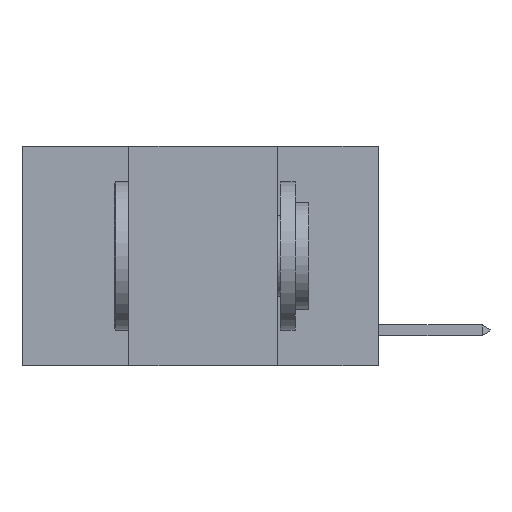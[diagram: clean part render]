
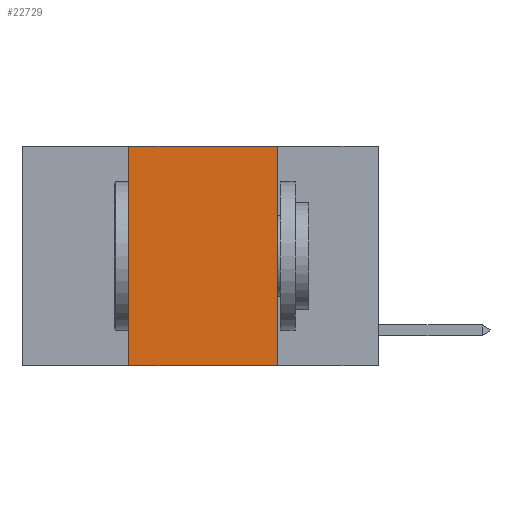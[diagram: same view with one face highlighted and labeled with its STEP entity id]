
A CAD part, left-side view. The second image highlights one B-rep face of the part: STEP entity #22729.
In plain terms, the highlighted planar face has unit normal (-1, 0, 0).
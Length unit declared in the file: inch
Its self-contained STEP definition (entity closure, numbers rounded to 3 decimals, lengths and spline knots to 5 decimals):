
#395 = DIRECTION ( 'NONE',  ( 0., 0., -1. ) ) ;
#428 = DIRECTION ( 'NONE',  ( 0., -1., 0. ) ) ;
#905 = VERTEX_POINT ( 'NONE', #9219 ) ;
#1697 = CARTESIAN_POINT ( 'NONE',  ( 0., 0.17, 0. ) ) ;
#2740 = VERTEX_POINT ( 'NONE', #23061 ) ;
#3685 = VECTOR ( 'NONE', #7489, 39.37008 ) ;
#4516 = PLANE ( 'NONE',  #23777 ) ;
#5400 = CARTESIAN_POINT ( 'NONE',  ( 0., 0.17, 0. ) ) ;
#5735 = ORIENTED_EDGE ( 'NONE', *, *, #16567, .F. ) ;
#7364 = DIRECTION ( 'NONE',  ( 0., -1., 0. ) ) ;
#7368 = ORIENTED_EDGE ( 'NONE', *, *, #22128, .T. ) ;
#7489 = DIRECTION ( 'NONE',  ( 0., 0., -1. ) ) ;
#9219 = CARTESIAN_POINT ( 'NONE',  ( 0., 0.17, -0.37 ) ) ;
#9378 = VECTOR ( 'NONE', #24487, 39.37008 ) ;
#10630 = VERTEX_POINT ( 'NONE', #1697 ) ;
#12193 = VERTEX_POINT ( 'NONE', #12789 ) ;
#12789 = CARTESIAN_POINT ( 'NONE',  ( 0., 0.42, -0.37 ) ) ;
#12941 = DIRECTION ( 'NONE',  ( 1., 0., 0. ) ) ;
#13678 = CARTESIAN_POINT ( 'NONE',  ( 0., 0.6, 0. ) ) ;
#15612 = LINE ( 'NONE', #22402, #9378 ) ;
#15742 = LINE ( 'NONE', #25429, #26122 ) ;
#16515 = ORIENTED_EDGE ( 'NONE', *, *, #19323, .F. ) ;
#16567 = EDGE_CURVE ( 'NONE', #10630, #905, #20302, .T. ) ;
#16672 = FACE_OUTER_BOUND ( 'NONE', #26459, .T. ) ;
#19323 = EDGE_CURVE ( 'NONE', #12193, #2740, #15612, .T. ) ;
#20302 = LINE ( 'NONE', #5400, #3685 ) ;
#22128 = EDGE_CURVE ( 'NONE', #12193, #905, #15742, .T. ) ;
#22402 = CARTESIAN_POINT ( 'NONE',  ( 0., 0.42, 0. ) ) ;
#22729 = ADVANCED_FACE ( 'NONE', ( #16672 ), #4516, .F. ) ;
#23061 = CARTESIAN_POINT ( 'NONE',  ( 0., 0.42, 0. ) ) ;
#23777 = AXIS2_PLACEMENT_3D ( 'NONE', #25398, #12941, #395 ) ;
#24321 = ORIENTED_EDGE ( 'NONE', *, *, #25746, .F. ) ;
#24487 = DIRECTION ( 'NONE',  ( 0., 0., 1. ) ) ;
#24615 = VECTOR ( 'NONE', #7364, 39.37008 ) ;
#25398 = CARTESIAN_POINT ( 'NONE',  ( 0., 0.6, 0. ) ) ;
#25429 = CARTESIAN_POINT ( 'NONE',  ( 0., 0.6, -0.37 ) ) ;
#25746 = EDGE_CURVE ( 'NONE', #2740, #10630, #25924, .T. ) ;
#25924 = LINE ( 'NONE', #13678, #24615 ) ;
#26122 = VECTOR ( 'NONE', #428, 39.37008 ) ;
#26459 = EDGE_LOOP ( 'NONE', ( #5735, #24321, #16515, #7368 ) ) ;
